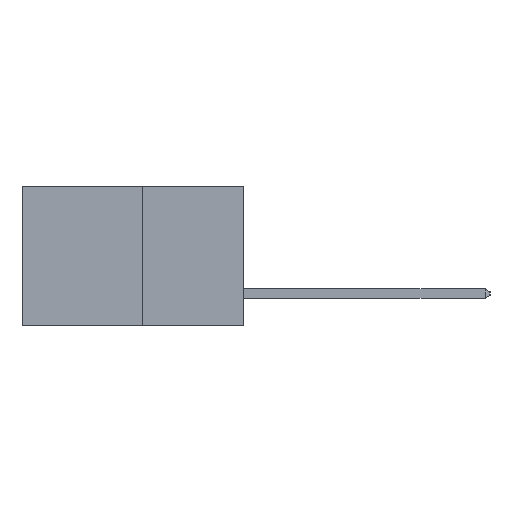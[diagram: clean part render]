
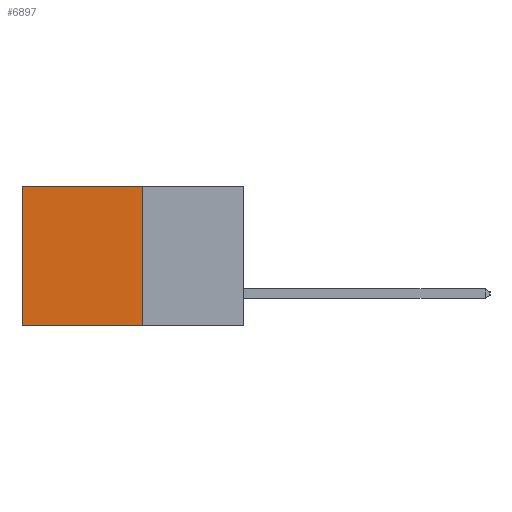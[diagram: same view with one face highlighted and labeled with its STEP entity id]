
A CAD part, left-side view. The second image highlights one B-rep face of the part: STEP entity #6897.
In plain terms, the highlighted planar face has unit normal (-1, 0, 0).
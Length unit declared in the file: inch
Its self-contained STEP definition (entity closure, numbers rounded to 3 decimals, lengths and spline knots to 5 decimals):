
#140 = ORIENTED_EDGE ( 'NONE', *, *, #6354, .T. ) ;
#534 = CARTESIAN_POINT ( 'NONE',  ( 0.277, 0.27, -0.37 ) ) ;
#633 = ORIENTED_EDGE ( 'NONE', *, *, #3139, .F. ) ;
#675 = VECTOR ( 'NONE', #3265, 39.37008 ) ;
#987 = VECTOR ( 'NONE', #7817, 39.37008 ) ;
#1275 = DIRECTION ( 'NONE',  ( 0., 0., -1. ) ) ;
#1432 = CARTESIAN_POINT ( 'NONE',  ( 0.277, 0.27, -0.37 ) ) ;
#1573 = AXIS2_PLACEMENT_3D ( 'NONE', #8455, #7700, #7594 ) ;
#2378 = LINE ( 'NONE', #1432, #12704 ) ;
#3139 = EDGE_CURVE ( 'NONE', #9026, #12147, #12215, .T. ) ;
#3200 = CARTESIAN_POINT ( 'NONE',  ( 0.277, 0.59, -0.37 ) ) ;
#3265 = DIRECTION ( 'NONE',  ( 0., 0., -1. ) ) ;
#3752 = CARTESIAN_POINT ( 'NONE',  ( 0.277, 0.27, -0.37 ) ) ;
#4822 = CARTESIAN_POINT ( 'NONE',  ( 0.277, 0.59, -0.37 ) ) ;
#6007 = EDGE_CURVE ( 'NONE', #7771, #12147, #8023, .T. ) ;
#6354 = EDGE_CURVE ( 'NONE', #12236, #7771, #9040, .T. ) ;
#6897 = ADVANCED_FACE ( 'NONE', ( #10122 ), #7865, .F. ) ;
#7594 = DIRECTION ( 'NONE',  ( 0., 0., -1. ) ) ;
#7700 = DIRECTION ( 'NONE',  ( 1., 0., 0. ) ) ;
#7771 = VERTEX_POINT ( 'NONE', #9200 ) ;
#7817 = DIRECTION ( 'NONE',  ( 0., 1., 0. ) ) ;
#7865 = PLANE ( 'NONE',  #1573 ) ;
#8023 = LINE ( 'NONE', #3200, #675 ) ;
#8203 = EDGE_CURVE ( 'NONE', #12236, #9026, #2378, .T. ) ;
#8263 = CARTESIAN_POINT ( 'NONE',  ( 0.277, 0.27, 0. ) ) ;
#8455 = CARTESIAN_POINT ( 'NONE',  ( 0.277, 0.27, -0.37 ) ) ;
#9026 = VERTEX_POINT ( 'NONE', #534 ) ;
#9040 = LINE ( 'NONE', #8263, #987 ) ;
#9200 = CARTESIAN_POINT ( 'NONE',  ( 0.277, 0.59, 0. ) ) ;
#9565 = VECTOR ( 'NONE', #12010, 39.37008 ) ;
#9625 = ORIENTED_EDGE ( 'NONE', *, *, #8203, .F. ) ;
#10106 = ORIENTED_EDGE ( 'NONE', *, *, #6007, .T. ) ;
#10122 = FACE_OUTER_BOUND ( 'NONE', #10786, .T. ) ;
#10786 = EDGE_LOOP ( 'NONE', ( #10106, #633, #9625, #140 ) ) ;
#12010 = DIRECTION ( 'NONE',  ( 0., 1., 0. ) ) ;
#12147 = VERTEX_POINT ( 'NONE', #4822 ) ;
#12215 = LINE ( 'NONE', #3752, #9565 ) ;
#12236 = VERTEX_POINT ( 'NONE', #12886 ) ;
#12704 = VECTOR ( 'NONE', #1275, 39.37008 ) ;
#12886 = CARTESIAN_POINT ( 'NONE',  ( 0.277, 0.27, 0. ) ) ;
